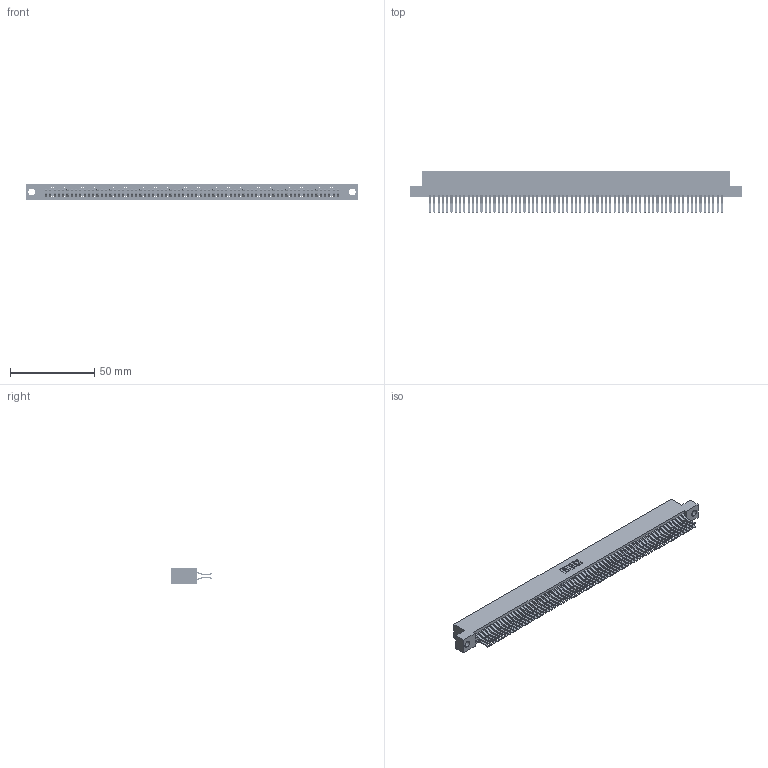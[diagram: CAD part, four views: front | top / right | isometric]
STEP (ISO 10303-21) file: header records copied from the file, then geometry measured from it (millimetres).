
FILE_DESCRIPTION (( 'STEP AP203' ), '1' );
FILE_NAME ('345-138-560-204.STEP', '2018-10-20T21:18:00', ( '' ), ( '' ), 'SwSTEP 2.0', 'SolidWorks 2016', '' );
FILE_SCHEMA (( 'CONFIG_CONTROL_DESIGN' ));
Length unit declared in the file: inch
Products named in the file (3): 345-138-560-204; 345-292-001_560 Tail; 345 Part_Flush Mounting Lugs - 0.156 Dia-TH
Assembly tree (139 placements, depth 2):
  345-138-560-204
    345 Part_Flush Mounting Lugs - 0.156 Dia-TH
    345-292-001_560 Tail  x138
Bounding box: 196.47 x 24.45 x 9.4 mm (x, y, z)
Volume: 20152.5 mm3; surface area: 32453.3 mm2
Topology: 139 solids, 139 shells, 7302 faces, 21731 edges, 14302 vertices
Faces by surface type: plane 4634, cylinder 2668
Entity records: 50595 total; most frequent: CARTESIAN_POINT 8456, ORIENTED_EDGE 8390, DIRECTION 7427, EDGE_CURVE 4195, LINE 3783, VECTOR 3783, VERTEX_POINT 2794, AXIS2_PLACEMENT_3D 1822
